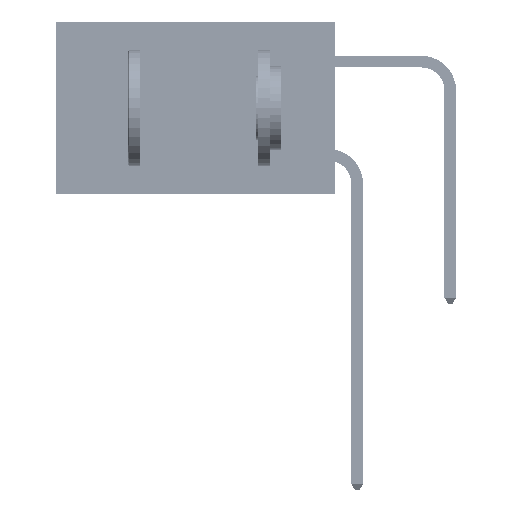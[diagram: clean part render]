
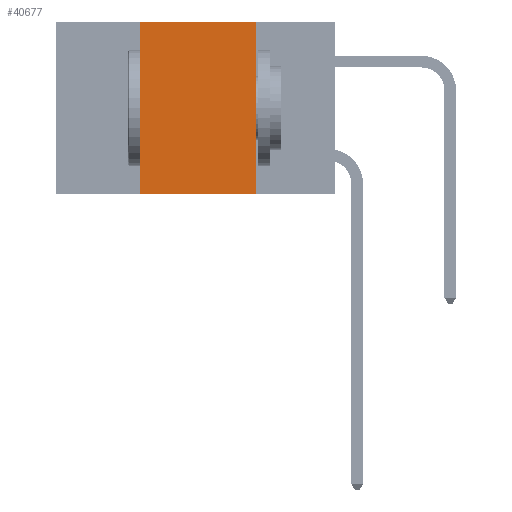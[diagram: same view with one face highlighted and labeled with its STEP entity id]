
A CAD part, left-side view. The second image highlights one B-rep face of the part: STEP entity #40677.
In plain terms, the highlighted planar face has unit normal (-1, 0, 0).
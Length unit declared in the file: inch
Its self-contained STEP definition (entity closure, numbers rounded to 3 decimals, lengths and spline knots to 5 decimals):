
#988 = LINE ( 'NONE', #41396, #46525 ) ;
#1091 = LINE ( 'NONE', #13947, #42302 ) ;
#1595 = DIRECTION ( 'NONE',  ( 0., -1., 0. ) ) ;
#2580 = VERTEX_POINT ( 'NONE', #51268 ) ;
#4315 = DIRECTION ( 'NONE',  ( 0., 0., -1. ) ) ;
#6167 = EDGE_LOOP ( 'NONE', ( #30083, #45855, #30689, #45686 ) ) ;
#6214 = EDGE_CURVE ( 'NONE', #25271, #2580, #988, .T. ) ;
#6975 = VERTEX_POINT ( 'NONE', #10073 ) ;
#9356 = VECTOR ( 'NONE', #34370, 39.37008 ) ;
#10073 = CARTESIAN_POINT ( 'NONE',  ( 0., 0.17, 0. ) ) ;
#12113 = EDGE_CURVE ( 'NONE', #6975, #2580, #41736, .T. ) ;
#13947 = CARTESIAN_POINT ( 'NONE',  ( 0., 0.42, 0. ) ) ;
#16827 = DIRECTION ( 'NONE',  ( 0., 0., -1. ) ) ;
#18164 = DIRECTION ( 'NONE',  ( 0., 0., 1. ) ) ;
#21216 = VECTOR ( 'NONE', #4315, 39.37008 ) ;
#21632 = EDGE_CURVE ( 'NONE', #25271, #38505, #1091, .T. ) ;
#25271 = VERTEX_POINT ( 'NONE', #48360 ) ;
#25397 = PLANE ( 'NONE',  #40493 ) ;
#30083 = ORIENTED_EDGE ( 'NONE', *, *, #12113, .F. ) ;
#30689 = ORIENTED_EDGE ( 'NONE', *, *, #21632, .F. ) ;
#32271 = CARTESIAN_POINT ( 'NONE',  ( 0., 0.17, 0. ) ) ;
#34033 = CARTESIAN_POINT ( 'NONE',  ( 0., 0.6, 0. ) ) ;
#34370 = DIRECTION ( 'NONE',  ( 0., -1., 0. ) ) ;
#38505 = VERTEX_POINT ( 'NONE', #50170 ) ;
#40493 = AXIS2_PLACEMENT_3D ( 'NONE', #45235, #41078, #16827 ) ;
#40677 = ADVANCED_FACE ( 'NONE', ( #41225 ), #25397, .F. ) ;
#41078 = DIRECTION ( 'NONE',  ( 1., 0., 0. ) ) ;
#41215 = LINE ( 'NONE', #34033, #9356 ) ;
#41225 = FACE_OUTER_BOUND ( 'NONE', #6167, .T. ) ;
#41396 = CARTESIAN_POINT ( 'NONE',  ( 0., 0.6, -0.37 ) ) ;
#41472 = EDGE_CURVE ( 'NONE', #38505, #6975, #41215, .T. ) ;
#41736 = LINE ( 'NONE', #32271, #21216 ) ;
#42302 = VECTOR ( 'NONE', #18164, 39.37008 ) ;
#45235 = CARTESIAN_POINT ( 'NONE',  ( 0., 0.6, 0. ) ) ;
#45686 = ORIENTED_EDGE ( 'NONE', *, *, #6214, .T. ) ;
#45855 = ORIENTED_EDGE ( 'NONE', *, *, #41472, .F. ) ;
#46525 = VECTOR ( 'NONE', #1595, 39.37008 ) ;
#48360 = CARTESIAN_POINT ( 'NONE',  ( 0., 0.42, -0.37 ) ) ;
#50170 = CARTESIAN_POINT ( 'NONE',  ( 0., 0.42, 0. ) ) ;
#51268 = CARTESIAN_POINT ( 'NONE',  ( 0., 0.17, -0.37 ) ) ;
